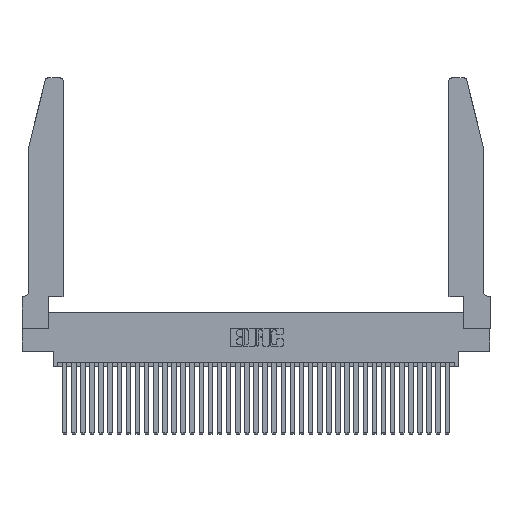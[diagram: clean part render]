
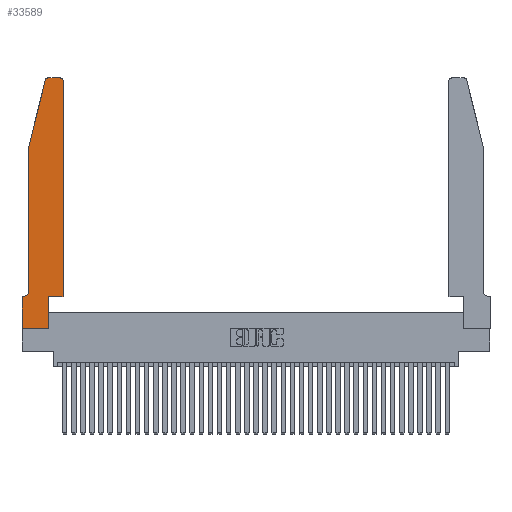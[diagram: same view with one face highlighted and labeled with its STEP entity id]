
A CAD part, top view. The second image highlights one B-rep face of the part: STEP entity #33589.
In plain terms, the highlighted planar face has unit normal (0, 0, 1).
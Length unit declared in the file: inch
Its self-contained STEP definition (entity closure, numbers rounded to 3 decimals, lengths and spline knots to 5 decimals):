
#80 = VECTOR ( 'NONE', #31638, 39.37008 ) ;
#151 = VECTOR ( 'NONE', #20206, 39.37008 ) ;
#564 = CARTESIAN_POINT ( 'NONE',  ( 0.2865, 0.35, 0.37 ) ) ;
#763 = DIRECTION ( 'NONE',  ( -1., 0., 0. ) ) ;
#2101 = LINE ( 'NONE', #11240, #10436 ) ;
#3093 = CARTESIAN_POINT ( 'NONE',  ( 0., 0., 0.37 ) ) ;
#3711 = CARTESIAN_POINT ( 'NONE',  ( 0.4505, 0.35, 0.37 ) ) ;
#3929 = EDGE_CURVE ( 'NONE', #20520, #35470, #9718, .T. ) ;
#4009 = CARTESIAN_POINT ( 'NONE',  ( 0.0055, 0.35, 0.37 ) ) ;
#4015 = DIRECTION ( 'NONE',  ( 0., 0., 1. ) ) ;
#4594 = LINE ( 'NONE', #32613, #8772 ) ;
#4973 = CARTESIAN_POINT ( 'NONE',  ( 0.4205, 2.75, 0.37 ) ) ;
#5373 = CARTESIAN_POINT ( 'NONE',  ( 0.4505, 0.35, 0.37 ) ) ;
#5986 = ORIENTED_EDGE ( 'NONE', *, *, #16788, .T. ) ;
#6029 = EDGE_CURVE ( 'NONE', #15868, #9214, #34145, .T. ) ;
#6484 = DIRECTION ( 'NONE',  ( 0., 0., -1. ) ) ;
#7480 = CARTESIAN_POINT ( 'NONE',  ( 0., 0.35, 0.37 ) ) ;
#7584 = CARTESIAN_POINT ( 'NONE',  ( 0.2865, 0.35, 0.37 ) ) ;
#7844 = CARTESIAN_POINT ( 'NONE',  ( 0.0755, 2., 0.37 ) ) ;
#7949 = EDGE_CURVE ( 'NONE', #8074, #13926, #2101, .T. ) ;
#8074 = VERTEX_POINT ( 'NONE', #4009 ) ;
#8184 = CIRCLE ( 'NONE', #27432, 0.03 ) ;
#8772 = VECTOR ( 'NONE', #14817, 39.37008 ) ;
#9149 = EDGE_CURVE ( 'NONE', #9214, #11674, #18675, .T. ) ;
#9207 = FACE_OUTER_BOUND ( 'NONE', #24396, .T. ) ;
#9214 = VERTEX_POINT ( 'NONE', #21396 ) ;
#9351 = LINE ( 'NONE', #11306, #26487 ) ;
#9553 = DIRECTION ( 'NONE',  ( 1., 0., 0. ) ) ;
#9646 = EDGE_CURVE ( 'NONE', #33163, #12409, #9351, .T. ) ;
#9718 = CIRCLE ( 'NONE', #33026, 0.03 ) ;
#10127 = EDGE_CURVE ( 'NONE', #27477, #33163, #13049, .T. ) ;
#10215 = DIRECTION ( 'NONE',  ( 0., 0., 1. ) ) ;
#10436 = VECTOR ( 'NONE', #30942, 39.37008 ) ;
#10595 = ORIENTED_EDGE ( 'NONE', *, *, #7949, .T. ) ;
#10604 = AXIS2_PLACEMENT_3D ( 'NONE', #15433, #6484, #763 ) ;
#10629 = VERTEX_POINT ( 'NONE', #27303 ) ;
#10778 = CARTESIAN_POINT ( 'NONE',  ( 0.2605, 2.75, 0.37 ) ) ;
#11240 = CARTESIAN_POINT ( 'NONE',  ( 0.0755, 0.35, 0.37 ) ) ;
#11277 = CARTESIAN_POINT ( 'NONE',  ( 0., 0., 0.37 ) ) ;
#11306 = CARTESIAN_POINT ( 'NONE',  ( 0.0755, 2., 0.37 ) ) ;
#11442 = DIRECTION ( 'NONE',  ( 0., -1., 0. ) ) ;
#11674 = VERTEX_POINT ( 'NONE', #7584 ) ;
#11708 = LINE ( 'NONE', #5373, #32909 ) ;
#12203 = VECTOR ( 'NONE', #12253, 39.37008 ) ;
#12253 = DIRECTION ( 'NONE',  ( 0., 1., 0. ) ) ;
#12409 = VERTEX_POINT ( 'NONE', #15130 ) ;
#12841 = VECTOR ( 'NONE', #21248, 39.37008 ) ;
#13049 = LINE ( 'NONE', #7844, #80 ) ;
#13148 = CARTESIAN_POINT ( 'NONE',  ( 0., 0., 0.37 ) ) ;
#13590 = ORIENTED_EDGE ( 'NONE', *, *, #6029, .T. ) ;
#13926 = VERTEX_POINT ( 'NONE', #7480 ) ;
#14255 = ORIENTED_EDGE ( 'NONE', *, *, #3929, .T. ) ;
#14817 = DIRECTION ( 'NONE',  ( 0., 1., 0. ) ) ;
#15130 = CARTESIAN_POINT ( 'NONE',  ( 0.0755, 0.42, 0.37 ) ) ;
#15433 = CARTESIAN_POINT ( 'NONE',  ( 0.0055, 0.42, 0.37 ) ) ;
#15447 = CARTESIAN_POINT ( 'NONE',  ( 0.0755, 2., 0.37 ) ) ;
#15868 = VERTEX_POINT ( 'NONE', #11277 ) ;
#15929 = CARTESIAN_POINT ( 'NONE',  ( 0.4205, 2.72, 0.37 ) ) ;
#16180 = CIRCLE ( 'NONE', #10604, 0.07 ) ;
#16788 = EDGE_CURVE ( 'NONE', #13926, #15868, #23660, .T. ) ;
#17236 = DIRECTION ( 'NONE',  ( 0., 0., 1. ) ) ;
#17781 = LINE ( 'NONE', #10778, #151 ) ;
#18075 = ORIENTED_EDGE ( 'NONE', *, *, #37439, .T. ) ;
#18675 = LINE ( 'NONE', #564, #12203 ) ;
#18973 = AXIS2_PLACEMENT_3D ( 'NONE', #26160, #17236, #26023 ) ;
#19638 = ORIENTED_EDGE ( 'NONE', *, *, #9646, .T. ) ;
#19932 = VECTOR ( 'NONE', #28223, 39.37008 ) ;
#20053 = VERTEX_POINT ( 'NONE', #3711 ) ;
#20206 = DIRECTION ( 'NONE',  ( -1., 0., 0. ) ) ;
#20520 = VERTEX_POINT ( 'NONE', #21078 ) ;
#21006 = ORIENTED_EDGE ( 'NONE', *, *, #25156, .T. ) ;
#21078 = CARTESIAN_POINT ( 'NONE',  ( 0.4505, 2.72, 0.37 ) ) ;
#21145 = CARTESIAN_POINT ( 'NONE',  ( 0.25487, 2.72718, 0.37 ) ) ;
#21248 = DIRECTION ( 'NONE',  ( 1., 0., 0. ) ) ;
#21396 = CARTESIAN_POINT ( 'NONE',  ( 0.2865, 0., 0.37 ) ) ;
#22983 = EDGE_CURVE ( 'NONE', #12409, #8074, #16180, .T. ) ;
#23660 = LINE ( 'NONE', #13148, #19932 ) ;
#24396 = EDGE_LOOP ( 'NONE', ( #29821, #21006, #34722, #19638, #37608, #10595, #5986, #13590, #33199, #32473, #18075, #14255 ) ) ;
#25156 = EDGE_CURVE ( 'NONE', #10629, #27477, #8184, .T. ) ;
#26023 = DIRECTION ( 'NONE',  ( 1., 0., 0. ) ) ;
#26160 = CARTESIAN_POINT ( 'NONE',  ( 0., 0.35, 0.37 ) ) ;
#26487 = VECTOR ( 'NONE', #11442, 39.37008 ) ;
#26742 = EDGE_CURVE ( 'NONE', #35470, #10629, #17781, .T. ) ;
#27303 = CARTESIAN_POINT ( 'NONE',  ( 0.284, 2.75, 0.37 ) ) ;
#27432 = AXIS2_PLACEMENT_3D ( 'NONE', #30476, #4015, #9553 ) ;
#27477 = VERTEX_POINT ( 'NONE', #21145 ) ;
#28223 = DIRECTION ( 'NONE',  ( 0., -1., 0. ) ) ;
#29224 = DIRECTION ( 'NONE',  ( 1., 0., 0. ) ) ;
#29821 = ORIENTED_EDGE ( 'NONE', *, *, #26742, .T. ) ;
#30476 = CARTESIAN_POINT ( 'NONE',  ( 0.284, 2.72, 0.37 ) ) ;
#30942 = DIRECTION ( 'NONE',  ( -1., 0., 0. ) ) ;
#31638 = DIRECTION ( 'NONE',  ( -0.239, -0.971, 0. ) ) ;
#32236 = EDGE_CURVE ( 'NONE', #11674, #20053, #11708, .T. ) ;
#32473 = ORIENTED_EDGE ( 'NONE', *, *, #32236, .T. ) ;
#32613 = CARTESIAN_POINT ( 'NONE',  ( 0.4505, 0.35, 0.37 ) ) ;
#32909 = VECTOR ( 'NONE', #29224, 39.37008 ) ;
#33026 = AXIS2_PLACEMENT_3D ( 'NONE', #15929, #10215, #36734 ) ;
#33163 = VERTEX_POINT ( 'NONE', #15447 ) ;
#33199 = ORIENTED_EDGE ( 'NONE', *, *, #9149, .T. ) ;
#33589 = ADVANCED_FACE ( 'NONE', ( #9207 ), #34950, .T. ) ;
#34145 = LINE ( 'NONE', #3093, #12841 ) ;
#34722 = ORIENTED_EDGE ( 'NONE', *, *, #10127, .T. ) ;
#34950 = PLANE ( 'NONE',  #18973 ) ;
#35470 = VERTEX_POINT ( 'NONE', #4973 ) ;
#36734 = DIRECTION ( 'NONE',  ( 1., 0., 0. ) ) ;
#37439 = EDGE_CURVE ( 'NONE', #20053, #20520, #4594, .T. ) ;
#37608 = ORIENTED_EDGE ( 'NONE', *, *, #22983, .T. ) ;
